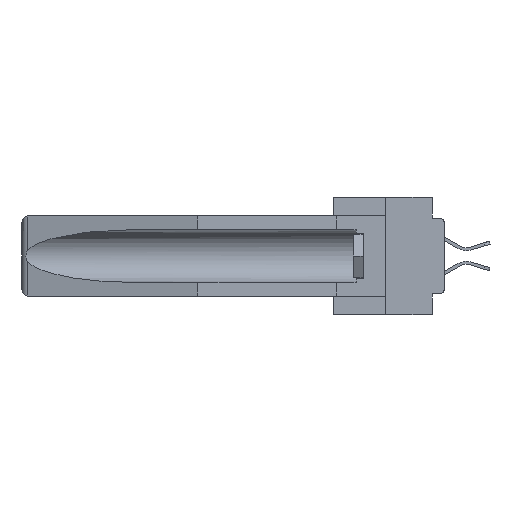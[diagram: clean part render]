
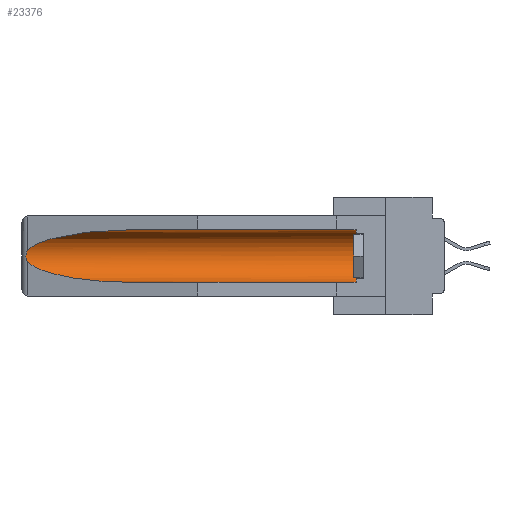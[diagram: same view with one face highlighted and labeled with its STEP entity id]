
A CAD part, left-side view. The second image highlights one B-rep face of the part: STEP entity #23376.
In plain terms, the highlighted cylindrical face has radius 2.857 mm (diameter 5.715 mm), a partial arc.
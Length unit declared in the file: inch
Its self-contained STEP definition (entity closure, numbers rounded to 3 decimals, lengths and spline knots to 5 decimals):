
#419 = CARTESIAN_POINT ( 'NONE',  ( 0.26537, 1.52718, -0.19328 ) ) ;
#1396 = CARTESIAN_POINT ( 'NONE',  ( 0.2673, 1.53269, -0.17917 ) ) ;
#1416 = EDGE_CURVE ( 'NONE', #24328, #29721, #10349, .T. ) ;
#3209 = VERTEX_POINT ( 'NONE', #27963 ) ;
#3894 = CARTESIAN_POINT ( 'NONE',  ( 0.155, -0.30754, -0.284 ) ) ;
#3901 = ORIENTED_EDGE ( 'NONE', *, *, #1416, .T. ) ;
#4931 = CARTESIAN_POINT ( 'NONE',  ( 0.25451, 1.48313, -0.24835 ) ) ;
#6527 = EDGE_LOOP ( 'NONE', ( #8508, #16094, #3901, #19269, #35520, #23131 ) ) ;
#7289 = CARTESIAN_POINT ( 'NONE',  ( 0.2675, 1.53308, -0.17534 ) ) ;
#7946 = CIRCLE ( 'NONE', #14045, 0.1125 ) ;
#8508 = ORIENTED_EDGE ( 'NONE', *, *, #16562, .T. ) ;
#9106 = CARTESIAN_POINT ( 'NONE',  ( 0.26537, 1.52718, -0.14972 ) ) ;
#9775 = CARTESIAN_POINT ( 'NONE',  ( 0.2673, 1.5327, -0.16383 ) ) ;
#10349 =( BOUNDED_CURVE ( )  B_SPLINE_CURVE ( 3, ( #36961, #4931, #10674, #36596 ),
 .UNSPECIFIED., .F., .F. ) 
 B_SPLINE_CURVE_WITH_KNOTS ( ( 4, 4 ),
 ( 0.1948, 1.5708 ),
 .UNSPECIFIED. ) 
 CURVE ( )  GEOMETRIC_REPRESENTATION_ITEM ( )  RATIONAL_B_SPLINE_CURVE ( ( 1., 0.848, 0.848, 1. ) ) 
 REPRESENTATION_ITEM ( '' )  );
#10370 = LINE ( 'NONE', #3894, #36916 ) ;
#10674 = CARTESIAN_POINT ( 'NONE',  ( 0.21114, 1.30732, -0.284 ) ) ;
#10694 = CARTESIAN_POINT ( 'NONE',  ( 0.21114, 1.30732, -0.059 ) ) ;
#10851 = CYLINDRICAL_SURFACE ( 'NONE', #22422, 0.1125 ) ;
#11029 = FACE_OUTER_BOUND ( 'NONE', #6527, .T. ) ;
#12486 = LINE ( 'NONE', #24053, #37337 ) ;
#12570 = B_SPLINE_CURVE_WITH_KNOTS ( 'NONE', 3,
 ( #27668, #21742, #13216, #9775, #36276, #7289, #1396, #21550, #33029, #19076 ),
 .UNSPECIFIED., .F., .F.,
 ( 4, 2, 2, 2, 4 ),
 ( 0., 0.00029, 0.00058, 0.00087, 0.00117 ),
 .UNSPECIFIED. ) ;
#13216 = CARTESIAN_POINT ( 'NONE',  ( 0.26654, 1.53092, -0.15636 ) ) ;
#13599 = CARTESIAN_POINT ( 'NONE',  ( 0.155, 0.126, -0.059 ) ) ;
#14045 = AXIS2_PLACEMENT_3D ( 'NONE', #19135, #27912, #33473 ) ;
#15138 = DIRECTION ( 'NONE',  ( 0., 1., 0. ) ) ;
#15513 = DIRECTION ( 'NONE',  ( 0., 1., 0. ) ) ;
#15597 = VERTEX_POINT ( 'NONE', #9106 ) ;
#16094 = ORIENTED_EDGE ( 'NONE', *, *, #22609, .T. ) ;
#16103 = EDGE_CURVE ( 'NONE', #34121, #35452, #12486, .T. ) ;
#16562 = EDGE_CURVE ( 'NONE', #35452, #15597, #32271, .T. ) ;
#19076 = CARTESIAN_POINT ( 'NONE',  ( 0.26537, 1.52718, -0.19328 ) ) ;
#19135 = CARTESIAN_POINT ( 'NONE',  ( 0.155, 0.126, -0.1715 ) ) ;
#19269 = ORIENTED_EDGE ( 'NONE', *, *, #33239, .F. ) ;
#21550 = CARTESIAN_POINT ( 'NONE',  ( 0.26655, 1.53094, -0.18657 ) ) ;
#21742 = CARTESIAN_POINT ( 'NONE',  ( 0.26597, 1.52961, -0.15275 ) ) ;
#22084 = CARTESIAN_POINT ( 'NONE',  ( 0.26537, 1.52718, -0.14972 ) ) ;
#22276 = CARTESIAN_POINT ( 'NONE',  ( 0.155, 1.07973, -0.059 ) ) ;
#22422 = AXIS2_PLACEMENT_3D ( 'NONE', #22425, #22611, #34293 ) ;
#22425 = CARTESIAN_POINT ( 'NONE',  ( 0.155, -0.30754, -0.1715 ) ) ;
#22455 = CARTESIAN_POINT ( 'NONE',  ( 0.25451, 1.48313, -0.09465 ) ) ;
#22609 = EDGE_CURVE ( 'NONE', #15597, #24328, #12570, .T. ) ;
#22611 = DIRECTION ( 'NONE',  ( 0., 1., 0. ) ) ;
#23131 = ORIENTED_EDGE ( 'NONE', *, *, #16103, .T. ) ;
#23376 = ADVANCED_FACE ( 'NONE', ( #11029 ), #10851, .F. ) ;
#24053 = CARTESIAN_POINT ( 'NONE',  ( 0.155, -0.30754, -0.059 ) ) ;
#24328 = VERTEX_POINT ( 'NONE', #419 ) ;
#25458 = EDGE_CURVE ( 'NONE', #3209, #34121, #7946, .T. ) ;
#27668 = CARTESIAN_POINT ( 'NONE',  ( 0.26537, 1.52718, -0.14972 ) ) ;
#27912 = DIRECTION ( 'NONE',  ( 0., -1., 0. ) ) ;
#27963 = CARTESIAN_POINT ( 'NONE',  ( 0.155, 0.126, -0.284 ) ) ;
#29721 = VERTEX_POINT ( 'NONE', #30056 ) ;
#30056 = CARTESIAN_POINT ( 'NONE',  ( 0.155, 1.07973, -0.284 ) ) ;
#30956 = CARTESIAN_POINT ( 'NONE',  ( 0.155, 1.07973, -0.059 ) ) ;
#32271 =( BOUNDED_CURVE ( )  B_SPLINE_CURVE ( 3, ( #22276, #10694, #22455, #22084 ),
 .UNSPECIFIED., .F., .F. ) 
 B_SPLINE_CURVE_WITH_KNOTS ( ( 4, 4 ),
 ( 4.71239, 6.08839 ),
 .UNSPECIFIED. ) 
 CURVE ( )  GEOMETRIC_REPRESENTATION_ITEM ( )  RATIONAL_B_SPLINE_CURVE ( ( 1., 0.848, 0.848, 1. ) ) 
 REPRESENTATION_ITEM ( '' )  );
#33029 = CARTESIAN_POINT ( 'NONE',  ( 0.26597, 1.5296, -0.19026 ) ) ;
#33239 = EDGE_CURVE ( 'NONE', #3209, #29721, #10370, .T. ) ;
#33473 = DIRECTION ( 'NONE',  ( 0., 0., 1. ) ) ;
#34121 = VERTEX_POINT ( 'NONE', #13599 ) ;
#34293 = DIRECTION ( 'NONE',  ( 0., 0., 1. ) ) ;
#35452 = VERTEX_POINT ( 'NONE', #30956 ) ;
#35520 = ORIENTED_EDGE ( 'NONE', *, *, #25458, .T. ) ;
#36276 = CARTESIAN_POINT ( 'NONE',  ( 0.2675, 1.53308, -0.16763 ) ) ;
#36596 = CARTESIAN_POINT ( 'NONE',  ( 0.155, 1.07973, -0.284 ) ) ;
#36916 = VECTOR ( 'NONE', #15513, 39.37008 ) ;
#36961 = CARTESIAN_POINT ( 'NONE',  ( 0.26537, 1.52718, -0.19328 ) ) ;
#37337 = VECTOR ( 'NONE', #15138, 39.37008 ) ;
